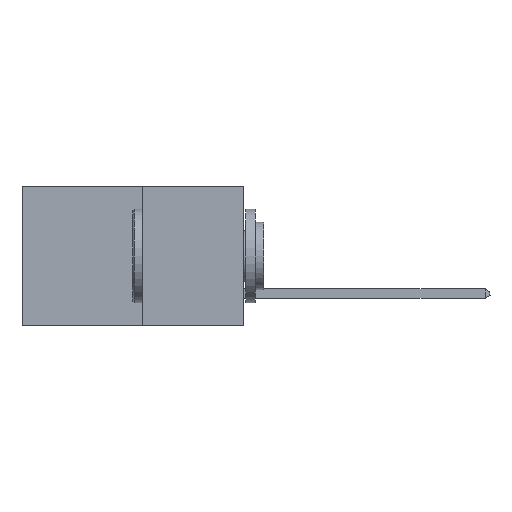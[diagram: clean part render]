
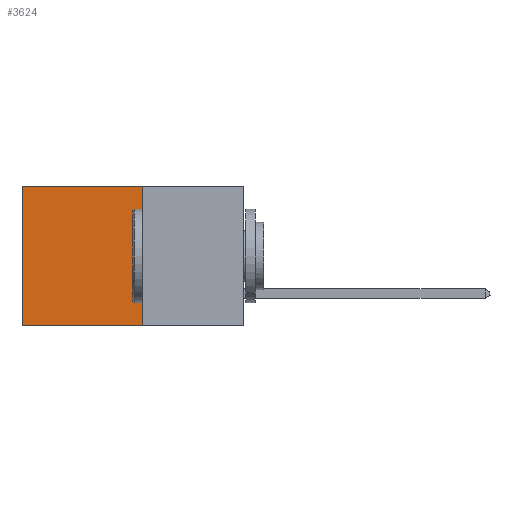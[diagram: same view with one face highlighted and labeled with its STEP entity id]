
A CAD part, left-side view. The second image highlights one B-rep face of the part: STEP entity #3624.
In plain terms, the highlighted planar face has unit normal (-1, 0, 0).
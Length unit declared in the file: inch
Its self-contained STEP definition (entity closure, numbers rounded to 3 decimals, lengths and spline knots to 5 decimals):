
#217 = LINE ( 'NONE', #9560, #2104 ) ;
#511 = CARTESIAN_POINT ( 'NONE',  ( 0.277, 0.27, -0.37 ) ) ;
#598 = DIRECTION ( 'NONE',  ( 0., 1., 0. ) ) ;
#742 = AXIS2_PLACEMENT_3D ( 'NONE', #11962, #11856, #11822 ) ;
#1873 = CARTESIAN_POINT ( 'NONE',  ( 0.277, 0.59, -0.37 ) ) ;
#1951 = ORIENTED_EDGE ( 'NONE', *, *, #6131, .F. ) ;
#2104 = VECTOR ( 'NONE', #9847, 39.37008 ) ;
#2473 = LINE ( 'NONE', #511, #7213 ) ;
#2608 = CARTESIAN_POINT ( 'NONE',  ( 0.277, 0.27, -0.37 ) ) ;
#3624 = ADVANCED_FACE ( 'NONE', ( #8298 ), #12009, .F. ) ;
#4055 = VECTOR ( 'NONE', #8894, 39.37008 ) ;
#4367 = LINE ( 'NONE', #9825, #4055 ) ;
#5214 = VERTEX_POINT ( 'NONE', #2608 ) ;
#5309 = EDGE_CURVE ( 'NONE', #5214, #6820, #2473, .T. ) ;
#6131 = EDGE_CURVE ( 'NONE', #11417, #5214, #9823, .T. ) ;
#6685 = ORIENTED_EDGE ( 'NONE', *, *, #5309, .F. ) ;
#6820 = VERTEX_POINT ( 'NONE', #1873 ) ;
#6899 = EDGE_LOOP ( 'NONE', ( #8908, #6685, #1951, #9490 ) ) ;
#6904 = CARTESIAN_POINT ( 'NONE',  ( 0.277, 0.59, 0. ) ) ;
#7103 = DIRECTION ( 'NONE',  ( 0., 0., -1. ) ) ;
#7141 = CARTESIAN_POINT ( 'NONE',  ( 0.277, 0.27, -0.37 ) ) ;
#7213 = VECTOR ( 'NONE', #598, 39.37008 ) ;
#7333 = VECTOR ( 'NONE', #7103, 39.37008 ) ;
#7515 = EDGE_CURVE ( 'NONE', #11417, #11308, #217, .T. ) ;
#8298 = FACE_OUTER_BOUND ( 'NONE', #6899, .T. ) ;
#8894 = DIRECTION ( 'NONE',  ( 0., 0., -1. ) ) ;
#8908 = ORIENTED_EDGE ( 'NONE', *, *, #10097, .T. ) ;
#8935 = CARTESIAN_POINT ( 'NONE',  ( 0.277, 0.27, 0. ) ) ;
#9490 = ORIENTED_EDGE ( 'NONE', *, *, #7515, .T. ) ;
#9560 = CARTESIAN_POINT ( 'NONE',  ( 0.277, 0.27, 0. ) ) ;
#9823 = LINE ( 'NONE', #7141, #7333 ) ;
#9825 = CARTESIAN_POINT ( 'NONE',  ( 0.277, 0.59, -0.37 ) ) ;
#9847 = DIRECTION ( 'NONE',  ( 0., 1., 0. ) ) ;
#10097 = EDGE_CURVE ( 'NONE', #11308, #6820, #4367, .T. ) ;
#11308 = VERTEX_POINT ( 'NONE', #6904 ) ;
#11417 = VERTEX_POINT ( 'NONE', #8935 ) ;
#11822 = DIRECTION ( 'NONE',  ( 0., 0., -1. ) ) ;
#11856 = DIRECTION ( 'NONE',  ( 1., 0., 0. ) ) ;
#11962 = CARTESIAN_POINT ( 'NONE',  ( 0.277, 0.27, -0.37 ) ) ;
#12009 = PLANE ( 'NONE',  #742 ) ;
